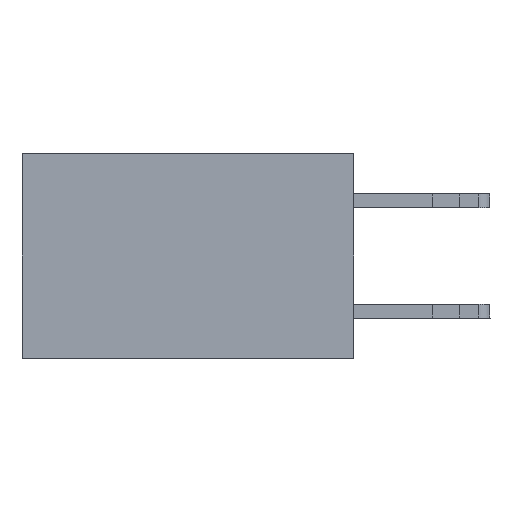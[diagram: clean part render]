
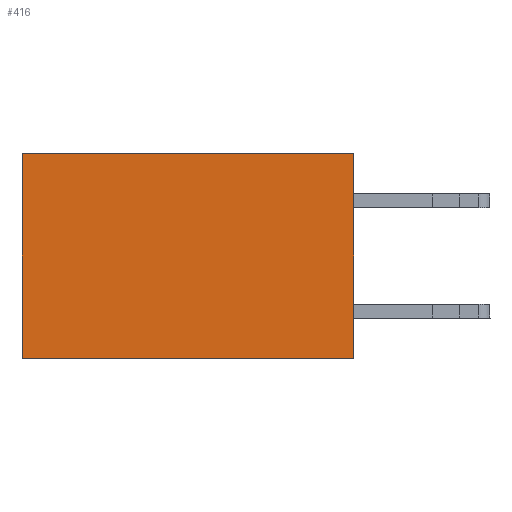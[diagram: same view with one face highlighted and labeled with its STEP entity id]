
A CAD part, left-side view. The second image highlights one B-rep face of the part: STEP entity #416.
In plain terms, the highlighted planar face has unit normal (-1, 0, 0).
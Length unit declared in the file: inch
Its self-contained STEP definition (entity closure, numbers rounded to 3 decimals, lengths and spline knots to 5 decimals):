
#416 = ADVANCED_FACE ( 'NONE', ( #10593 ), #20094, .F. ) ;
#664 = AXIS2_PLACEMENT_3D ( 'NONE', #19935, #19902, #19876 ) ;
#1509 = EDGE_LOOP ( 'NONE', ( #10089, #14340, #15721, #14261 ) ) ;
#3077 = CARTESIAN_POINT ( 'NONE',  ( 0.2875, 0., -0.37 ) ) ;
#3149 = LINE ( 'NONE', #16569, #20674 ) ;
#5284 = EDGE_CURVE ( 'NONE', #22600, #6943, #19411, .T. ) ;
#5482 = VECTOR ( 'NONE', #11885, 39.37008 ) ;
#6347 = VECTOR ( 'NONE', #10008, 39.37008 ) ;
#6551 = CARTESIAN_POINT ( 'NONE',  ( 0.2875, 0., 0. ) ) ;
#6943 = VERTEX_POINT ( 'NONE', #19788 ) ;
#9138 = DIRECTION ( 'NONE',  ( 0., 0., -1. ) ) ;
#10008 = DIRECTION ( 'NONE',  ( 0., 1., 0. ) ) ;
#10059 = VERTEX_POINT ( 'NONE', #10583 ) ;
#10089 = ORIENTED_EDGE ( 'NONE', *, *, #22172, .T. ) ;
#10583 = CARTESIAN_POINT ( 'NONE',  ( 0.2875, 0.6, 0. ) ) ;
#10593 = FACE_OUTER_BOUND ( 'NONE', #1509, .T. ) ;
#10990 = EDGE_CURVE ( 'NONE', #16453, #22600, #3149, .T. ) ;
#11599 = LINE ( 'NONE', #6551, #6347 ) ;
#11885 = DIRECTION ( 'NONE',  ( 0., 1., 0. ) ) ;
#14261 = ORIENTED_EDGE ( 'NONE', *, *, #19459, .T. ) ;
#14340 = ORIENTED_EDGE ( 'NONE', *, *, #5284, .F. ) ;
#14346 = LINE ( 'NONE', #19568, #19533 ) ;
#15721 = ORIENTED_EDGE ( 'NONE', *, *, #10990, .F. ) ;
#16453 = VERTEX_POINT ( 'NONE', #21753 ) ;
#16569 = CARTESIAN_POINT ( 'NONE',  ( 0.2875, 0., 0. ) ) ;
#18285 = DIRECTION ( 'NONE',  ( 0., 0., -1. ) ) ;
#19411 = LINE ( 'NONE', #22200, #5482 ) ;
#19459 = EDGE_CURVE ( 'NONE', #16453, #10059, #11599, .T. ) ;
#19533 = VECTOR ( 'NONE', #9138, 39.37008 ) ;
#19568 = CARTESIAN_POINT ( 'NONE',  ( 0.2875, 0.6, 0. ) ) ;
#19788 = CARTESIAN_POINT ( 'NONE',  ( 0.2875, 0.6, -0.37 ) ) ;
#19876 = DIRECTION ( 'NONE',  ( 0., 0., -1. ) ) ;
#19902 = DIRECTION ( 'NONE',  ( 1., 0., 0. ) ) ;
#19935 = CARTESIAN_POINT ( 'NONE',  ( 0.2875, 0., 0. ) ) ;
#20094 = PLANE ( 'NONE',  #664 ) ;
#20674 = VECTOR ( 'NONE', #18285, 39.37008 ) ;
#21753 = CARTESIAN_POINT ( 'NONE',  ( 0.2875, 0., 0. ) ) ;
#22172 = EDGE_CURVE ( 'NONE', #10059, #6943, #14346, .T. ) ;
#22200 = CARTESIAN_POINT ( 'NONE',  ( 0.2875, 0., -0.37 ) ) ;
#22600 = VERTEX_POINT ( 'NONE', #3077 ) ;
